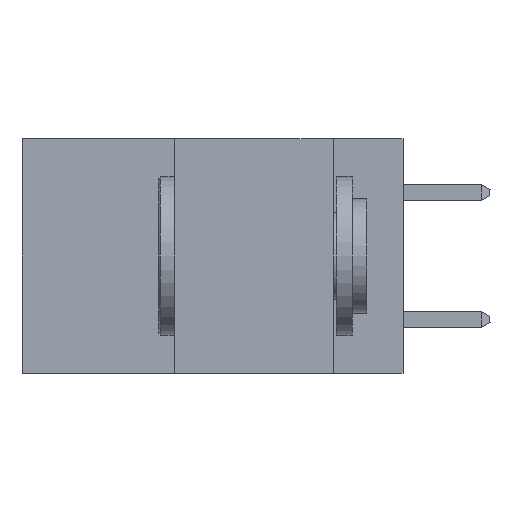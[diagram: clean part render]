
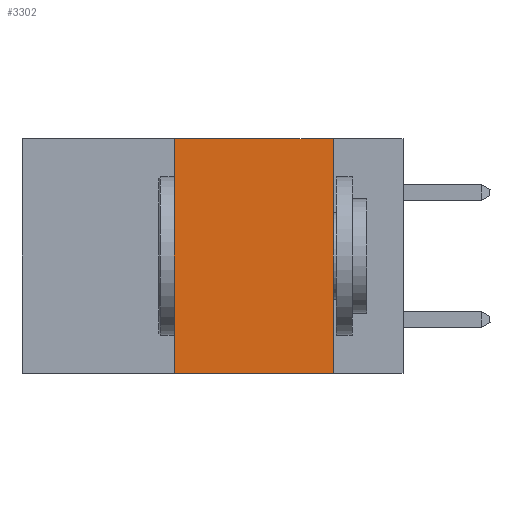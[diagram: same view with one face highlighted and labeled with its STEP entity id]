
A CAD part, left-side view. The second image highlights one B-rep face of the part: STEP entity #3302.
In plain terms, the highlighted planar face has unit normal (-1, 0, 0).
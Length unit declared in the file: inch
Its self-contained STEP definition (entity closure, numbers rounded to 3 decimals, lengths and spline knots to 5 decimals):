
#216 = CARTESIAN_POINT ( 'NONE',  ( 0., 0.6, 0. ) ) ;
#987 = VECTOR ( 'NONE', #19854, 39.37008 ) ;
#2013 = CARTESIAN_POINT ( 'NONE',  ( 0., 0.6, -0.37 ) ) ;
#2266 = ORIENTED_EDGE ( 'NONE', *, *, #22323, .T. ) ;
#2819 = VECTOR ( 'NONE', #10812, 39.37008 ) ;
#3302 = ADVANCED_FACE ( 'NONE', ( #20290 ), #20080, .F. ) ;
#5694 = DIRECTION ( 'NONE',  ( 0., 0., -1. ) ) ;
#6903 = EDGE_LOOP ( 'NONE', ( #15873, #11218, #14935, #2266 ) ) ;
#7177 = CARTESIAN_POINT ( 'NONE',  ( 0., 0.36, 0. ) ) ;
#7671 = VERTEX_POINT ( 'NONE', #19757 ) ;
#8265 = AXIS2_PLACEMENT_3D ( 'NONE', #216, #16730, #5694 ) ;
#8416 = CARTESIAN_POINT ( 'NONE',  ( 0., 0.36, 0. ) ) ;
#9250 = LINE ( 'NONE', #2013, #10136 ) ;
#9695 = EDGE_CURVE ( 'NONE', #17935, #14130, #13878, .T. ) ;
#10059 = CARTESIAN_POINT ( 'NONE',  ( 0., 0.11, 0. ) ) ;
#10136 = VECTOR ( 'NONE', #18184, 39.37008 ) ;
#10164 = DIRECTION ( 'NONE',  ( 0., 0., -1. ) ) ;
#10812 = DIRECTION ( 'NONE',  ( 0., 0., 1. ) ) ;
#11218 = ORIENTED_EDGE ( 'NONE', *, *, #17125, .F. ) ;
#11254 = LINE ( 'NONE', #7177, #2819 ) ;
#11387 = LINE ( 'NONE', #12614, #987 ) ;
#12614 = CARTESIAN_POINT ( 'NONE',  ( 0., 0.6, 0. ) ) ;
#13878 = LINE ( 'NONE', #20942, #18098 ) ;
#14130 = VERTEX_POINT ( 'NONE', #21491 ) ;
#14935 = ORIENTED_EDGE ( 'NONE', *, *, #21516, .F. ) ;
#15873 = ORIENTED_EDGE ( 'NONE', *, *, #9695, .F. ) ;
#16730 = DIRECTION ( 'NONE',  ( 1., 0., 0. ) ) ;
#17125 = EDGE_CURVE ( 'NONE', #20681, #17935, #11387, .T. ) ;
#17935 = VERTEX_POINT ( 'NONE', #10059 ) ;
#18098 = VECTOR ( 'NONE', #10164, 39.37008 ) ;
#18184 = DIRECTION ( 'NONE',  ( 0., -1., 0. ) ) ;
#19757 = CARTESIAN_POINT ( 'NONE',  ( 0., 0.36, -0.37 ) ) ;
#19854 = DIRECTION ( 'NONE',  ( 0., -1., 0. ) ) ;
#20080 = PLANE ( 'NONE',  #8265 ) ;
#20290 = FACE_OUTER_BOUND ( 'NONE', #6903, .T. ) ;
#20681 = VERTEX_POINT ( 'NONE', #8416 ) ;
#20942 = CARTESIAN_POINT ( 'NONE',  ( 0., 0.11, 0. ) ) ;
#21491 = CARTESIAN_POINT ( 'NONE',  ( 0., 0.11, -0.37 ) ) ;
#21516 = EDGE_CURVE ( 'NONE', #7671, #20681, #11254, .T. ) ;
#22323 = EDGE_CURVE ( 'NONE', #7671, #14130, #9250, .T. ) ;
